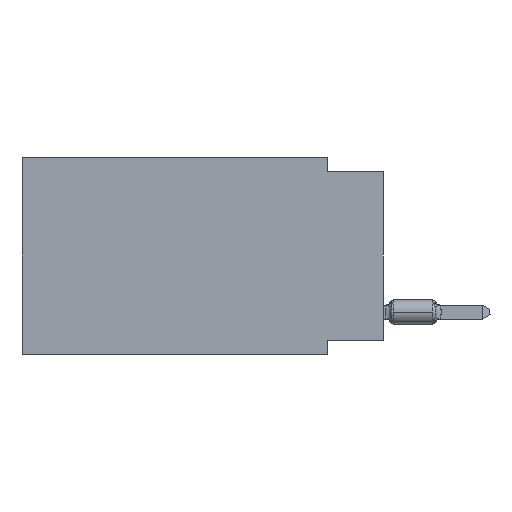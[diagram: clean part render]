
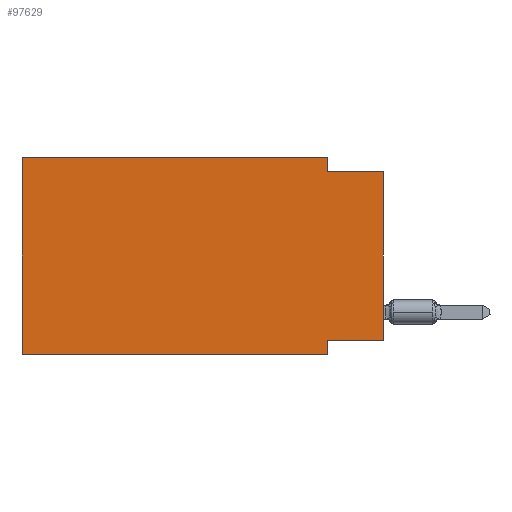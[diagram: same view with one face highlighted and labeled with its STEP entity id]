
A CAD part, left-side view. The second image highlights one B-rep face of the part: STEP entity #97629.
In plain terms, the highlighted planar face has unit normal (-1, 0, 0).
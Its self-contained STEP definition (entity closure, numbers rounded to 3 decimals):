
#276 = DIRECTION ( 'NONE',  ( 0., -1., 0. ) ) ;
#369 = DIRECTION ( 'NONE',  ( 0., 0., 1. ) ) ;
#473 = VERTEX_POINT ( 'NONE', #9774 ) ;
#998 = ORIENTED_EDGE ( 'NONE', *, *, #66108, .F. ) ;
#4628 = DIRECTION ( 'NONE',  ( 0., -1., 0. ) ) ;
#5098 = ORIENTED_EDGE ( 'NONE', *, *, #7435, .T. ) ;
#5985 = DIRECTION ( 'NONE',  ( 0., 0., -1. ) ) ;
#6975 = CARTESIAN_POINT ( 'NONE',  ( 0., 16.383, -8.89 ) ) ;
#7239 = VECTOR ( 'NONE', #66385, 1000. ) ;
#7435 = EDGE_CURVE ( 'NONE', #87294, #21933, #93636, .T. ) ;
#7441 = CARTESIAN_POINT ( 'NONE',  ( 0., 2.54, 0. ) ) ;
#9774 = CARTESIAN_POINT ( 'NONE',  ( 0., 2.54, -0.635 ) ) ;
#11096 = VECTOR ( 'NONE', #276, 1000. ) ;
#13517 = VERTEX_POINT ( 'NONE', #7441 ) ;
#14266 = EDGE_CURVE ( 'NONE', #473, #61287, #72940, .T. ) ;
#15279 = DIRECTION ( 'NONE',  ( 0., -1., 0. ) ) ;
#19151 = LINE ( 'NONE', #50813, #7239 ) ;
#21154 = EDGE_LOOP ( 'NONE', ( #100087, #42096, #76469, #72354, #35301, #5098, #80558, #998 ) ) ;
#21933 = VERTEX_POINT ( 'NONE', #55837 ) ;
#24354 = CARTESIAN_POINT ( 'NONE',  ( 0., 16.383, 0. ) ) ;
#25939 = CARTESIAN_POINT ( 'NONE',  ( 0., 2.54, 0. ) ) ;
#26237 = CARTESIAN_POINT ( 'NONE',  ( 0., 0., -8.255 ) ) ;
#30369 = DIRECTION ( 'NONE',  ( 1., 0., 0. ) ) ;
#31506 = VERTEX_POINT ( 'NONE', #24354 ) ;
#32548 = VECTOR ( 'NONE', #66701, 1000. ) ;
#34059 = PLANE ( 'NONE',  #102247 ) ;
#35301 = ORIENTED_EDGE ( 'NONE', *, *, #73860, .F. ) ;
#42096 = ORIENTED_EDGE ( 'NONE', *, *, #14266, .F. ) ;
#44079 = LINE ( 'NONE', #75736, #45101 ) ;
#45101 = VECTOR ( 'NONE', #4628, 1000. ) ;
#47089 = LINE ( 'NONE', #102625, #98756 ) ;
#50813 = CARTESIAN_POINT ( 'NONE',  ( 0., 0., 0. ) ) ;
#55837 = CARTESIAN_POINT ( 'NONE',  ( 0., 2.54, -8.89 ) ) ;
#56542 = VERTEX_POINT ( 'NONE', #98939 ) ;
#59145 = DIRECTION ( 'NONE',  ( 0., 0., -1. ) ) ;
#59176 = EDGE_CURVE ( 'NONE', #31506, #13517, #44079, .T. ) ;
#60783 = EDGE_CURVE ( 'NONE', #82413, #61287, #19151, .T. ) ;
#61287 = VERTEX_POINT ( 'NONE', #66766 ) ;
#62200 = CARTESIAN_POINT ( 'NONE',  ( 0., 16.383, 0. ) ) ;
#65207 = DIRECTION ( 'NONE',  ( 0., 0., -1. ) ) ;
#66108 = EDGE_CURVE ( 'NONE', #82413, #56542, #81234, .T. ) ;
#66385 = DIRECTION ( 'NONE',  ( 0., 0., 1. ) ) ;
#66701 = DIRECTION ( 'NONE',  ( 0., 1., 0. ) ) ;
#66766 = CARTESIAN_POINT ( 'NONE',  ( 0., 0., -0.635 ) ) ;
#71411 = CARTESIAN_POINT ( 'NONE',  ( 0., 0., -0.635 ) ) ;
#72354 = ORIENTED_EDGE ( 'NONE', *, *, #59176, .F. ) ;
#72940 = LINE ( 'NONE', #71411, #11096 ) ;
#73781 = VECTOR ( 'NONE', #15279, 1000. ) ;
#73860 = EDGE_CURVE ( 'NONE', #87294, #31506, #101628, .T. ) ;
#75085 = VECTOR ( 'NONE', #369, 1000. ) ;
#75736 = CARTESIAN_POINT ( 'NONE',  ( 0., 16.383, 0. ) ) ;
#76469 = ORIENTED_EDGE ( 'NONE', *, *, #77717, .F. ) ;
#76529 = CARTESIAN_POINT ( 'NONE',  ( 0., 16.383, -8.89 ) ) ;
#77717 = EDGE_CURVE ( 'NONE', #13517, #473, #82469, .T. ) ;
#80404 = VECTOR ( 'NONE', #59145, 1000. ) ;
#80558 = ORIENTED_EDGE ( 'NONE', *, *, #96146, .F. ) ;
#81234 = LINE ( 'NONE', #26237, #32548 ) ;
#82413 = VERTEX_POINT ( 'NONE', #88883 ) ;
#82469 = LINE ( 'NONE', #25939, #80404 ) ;
#87294 = VERTEX_POINT ( 'NONE', #6975 ) ;
#88883 = CARTESIAN_POINT ( 'NONE',  ( 0., 0., -8.255 ) ) ;
#91631 = FACE_OUTER_BOUND ( 'NONE', #21154, .T. ) ;
#92151 = CARTESIAN_POINT ( 'NONE',  ( 0., 16.383, 0. ) ) ;
#93636 = LINE ( 'NONE', #76529, #73781 ) ;
#96146 = EDGE_CURVE ( 'NONE', #56542, #21933, #47089, .T. ) ;
#97629 = ADVANCED_FACE ( 'NONE', ( #91631 ), #34059, .F. ) ;
#98756 = VECTOR ( 'NONE', #65207, 1000. ) ;
#98939 = CARTESIAN_POINT ( 'NONE',  ( 0., 2.54, -8.255 ) ) ;
#100087 = ORIENTED_EDGE ( 'NONE', *, *, #60783, .T. ) ;
#101628 = LINE ( 'NONE', #62200, #75085 ) ;
#102247 = AXIS2_PLACEMENT_3D ( 'NONE', #92151, #30369, #5985 ) ;
#102625 = CARTESIAN_POINT ( 'NONE',  ( 0., 2.54, -8.89 ) ) ;
